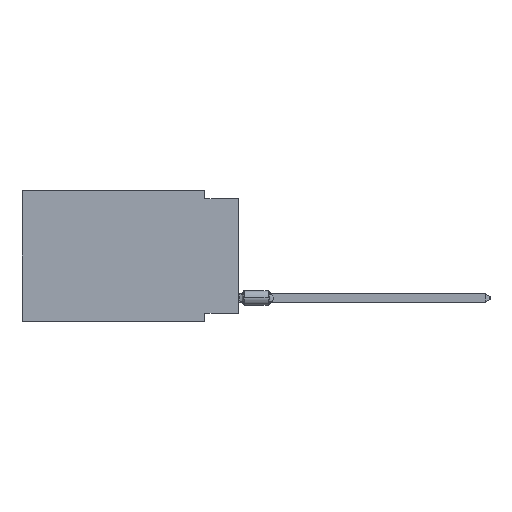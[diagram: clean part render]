
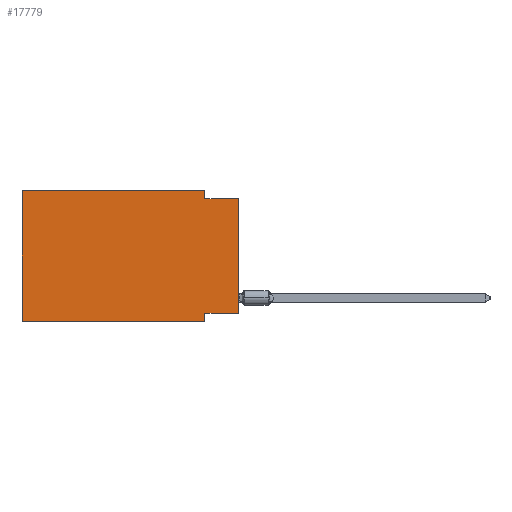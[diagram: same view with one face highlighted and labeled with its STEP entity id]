
A CAD part, left-side view. The second image highlights one B-rep face of the part: STEP entity #17779.
In plain terms, the highlighted planar face has unit normal (-1, 0, 0).
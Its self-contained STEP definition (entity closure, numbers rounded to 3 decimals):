
#258 = CARTESIAN_POINT ( 'NONE',  ( 0., 16.383, -9.906 ) ) ;
#559 = EDGE_CURVE ( 'NONE', #36244, #25270, #10685, .T. ) ;
#605 = CARTESIAN_POINT ( 'NONE',  ( 0., 0., 0. ) ) ;
#627 = DIRECTION ( 'NONE',  ( 0., 0., -1. ) ) ;
#719 = LINE ( 'NONE', #10592, #30217 ) ;
#1408 = VECTOR ( 'NONE', #627, 1000. ) ;
#3758 = EDGE_CURVE ( 'NONE', #21663, #36244, #719, .T. ) ;
#3973 = DIRECTION ( 'NONE',  ( 0., 0., -1. ) ) ;
#6046 = PLANE ( 'NONE',  #12944 ) ;
#6178 = CARTESIAN_POINT ( 'NONE',  ( 0., 0., -9.271 ) ) ;
#6231 = DIRECTION ( 'NONE',  ( 0., -1., 0. ) ) ;
#6326 = ORIENTED_EDGE ( 'NONE', *, *, #11031, .T. ) ;
#6330 = VECTOR ( 'NONE', #21187, 1000. ) ;
#6862 = ORIENTED_EDGE ( 'NONE', *, *, #24539, .F. ) ;
#9173 = LINE ( 'NONE', #11714, #6330 ) ;
#9500 = CARTESIAN_POINT ( 'NONE',  ( 0., 2.54, -9.906 ) ) ;
#10311 = LINE ( 'NONE', #32412, #21631 ) ;
#10592 = CARTESIAN_POINT ( 'NONE',  ( 0., 16.383, 0. ) ) ;
#10643 = ORIENTED_EDGE ( 'NONE', *, *, #40026, .F. ) ;
#10685 = LINE ( 'NONE', #26916, #25990 ) ;
#11031 = EDGE_CURVE ( 'NONE', #39003, #24214, #39280, .T. ) ;
#11714 = CARTESIAN_POINT ( 'NONE',  ( 0., 0., -0.635 ) ) ;
#12130 = DIRECTION ( 'NONE',  ( 1., 0., 0. ) ) ;
#12770 = CARTESIAN_POINT ( 'NONE',  ( 0., 2.54, -9.271 ) ) ;
#12944 = AXIS2_PLACEMENT_3D ( 'NONE', #22251, #12130, #41329 ) ;
#13152 = LINE ( 'NONE', #25194, #16780 ) ;
#13871 = CARTESIAN_POINT ( 'NONE',  ( 0., 2.54, -9.906 ) ) ;
#14301 = EDGE_LOOP ( 'NONE', ( #6326, #6862, #41325, #36993, #37312, #20415, #10643, #31344 ) ) ;
#15725 = VERTEX_POINT ( 'NONE', #12770 ) ;
#16310 = CARTESIAN_POINT ( 'NONE',  ( 0., 0., -9.271 ) ) ;
#16780 = VECTOR ( 'NONE', #6231, 1000. ) ;
#17779 = ADVANCED_FACE ( 'NONE', ( #38612 ), #6046, .F. ) ;
#20415 = ORIENTED_EDGE ( 'NONE', *, *, #39012, .T. ) ;
#21187 = DIRECTION ( 'NONE',  ( 0., -1., 0. ) ) ;
#21631 = VECTOR ( 'NONE', #23167, 1000. ) ;
#21663 = VERTEX_POINT ( 'NONE', #29739 ) ;
#22224 = CARTESIAN_POINT ( 'NONE',  ( 0., 2.54, -0.635 ) ) ;
#22251 = CARTESIAN_POINT ( 'NONE',  ( 0., 16.383, 0. ) ) ;
#23008 = LINE ( 'NONE', #6178, #32910 ) ;
#23167 = DIRECTION ( 'NONE',  ( 0., 0., 1. ) ) ;
#23388 = EDGE_CURVE ( 'NONE', #31125, #21663, #10311, .T. ) ;
#24214 = VERTEX_POINT ( 'NONE', #40779 ) ;
#24539 = EDGE_CURVE ( 'NONE', #25270, #24214, #9173, .T. ) ;
#25161 = CARTESIAN_POINT ( 'NONE',  ( 0., 2.54, 0. ) ) ;
#25194 = CARTESIAN_POINT ( 'NONE',  ( 0., 16.383, -9.906 ) ) ;
#25270 = VERTEX_POINT ( 'NONE', #22224 ) ;
#25990 = VECTOR ( 'NONE', #3973, 1000. ) ;
#26154 = DIRECTION ( 'NONE',  ( 0., 1., 0. ) ) ;
#26916 = CARTESIAN_POINT ( 'NONE',  ( 0., 2.54, 0. ) ) ;
#28017 = EDGE_CURVE ( 'NONE', #39003, #15725, #23008, .T. ) ;
#29739 = CARTESIAN_POINT ( 'NONE',  ( 0., 16.383, 0. ) ) ;
#30217 = VECTOR ( 'NONE', #36037, 1000. ) ;
#30520 = VECTOR ( 'NONE', #39695, 1000. ) ;
#31125 = VERTEX_POINT ( 'NONE', #258 ) ;
#31344 = ORIENTED_EDGE ( 'NONE', *, *, #28017, .F. ) ;
#32412 = CARTESIAN_POINT ( 'NONE',  ( 0., 16.383, 0. ) ) ;
#32910 = VECTOR ( 'NONE', #26154, 1000. ) ;
#36037 = DIRECTION ( 'NONE',  ( 0., -1., 0. ) ) ;
#36244 = VERTEX_POINT ( 'NONE', #25161 ) ;
#36780 = VERTEX_POINT ( 'NONE', #9500 ) ;
#36993 = ORIENTED_EDGE ( 'NONE', *, *, #3758, .F. ) ;
#37312 = ORIENTED_EDGE ( 'NONE', *, *, #23388, .F. ) ;
#38612 = FACE_OUTER_BOUND ( 'NONE', #14301, .T. ) ;
#38887 = LINE ( 'NONE', #13871, #1408 ) ;
#39003 = VERTEX_POINT ( 'NONE', #16310 ) ;
#39012 = EDGE_CURVE ( 'NONE', #31125, #36780, #13152, .T. ) ;
#39280 = LINE ( 'NONE', #605, #30520 ) ;
#39695 = DIRECTION ( 'NONE',  ( 0., 0., 1. ) ) ;
#40026 = EDGE_CURVE ( 'NONE', #15725, #36780, #38887, .T. ) ;
#40779 = CARTESIAN_POINT ( 'NONE',  ( 0., 0., -0.635 ) ) ;
#41325 = ORIENTED_EDGE ( 'NONE', *, *, #559, .F. ) ;
#41329 = DIRECTION ( 'NONE',  ( 0., 0., -1. ) ) ;
